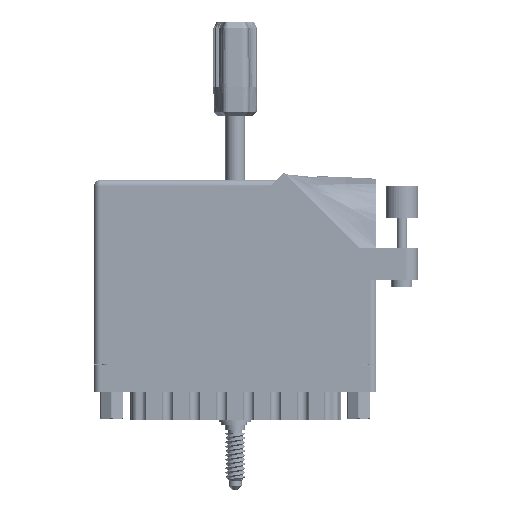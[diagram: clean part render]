
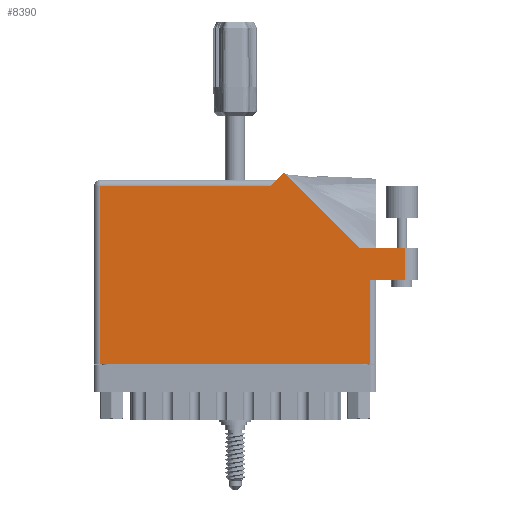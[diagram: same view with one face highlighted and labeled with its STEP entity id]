
A CAD part, front view. The second image highlights one B-rep face of the part: STEP entity #8390.
In plain terms, the highlighted face is planar.
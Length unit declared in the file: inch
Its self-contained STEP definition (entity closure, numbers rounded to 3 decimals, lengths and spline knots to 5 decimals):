
#1445 = ORIENTED_EDGE ( 'NONE', *, *, #68756, .T. ) ;
#1887 = CARTESIAN_POINT ( 'NONE',  ( 2.656, 0.815, 0. ) ) ;
#2625 = EDGE_CURVE ( 'NONE', #33896, #48656, #38547, .T. ) ;
#3944 = ORIENTED_EDGE ( 'NONE', *, *, #40752, .T. ) ;
#4784 = CARTESIAN_POINT ( 'NONE',  ( 3.118, 1.122, 0. ) ) ;
#5384 = DIRECTION ( 'NONE',  ( 0., 0., -1. ) ) ;
#8390 = ADVANCED_FACE ( 'NONE', ( #10046 ), #50888, .F. ) ;
#9209 = VECTOR ( 'NONE', #99094, 39.37008 ) ;
#10046 = FACE_OUTER_BOUND ( 'NONE', #59269, .T. ) ;
#10712 = LINE ( 'NONE', #1887, #82452 ) ;
#11647 = ORIENTED_EDGE ( 'NONE', *, *, #65456, .T. ) ;
#11669 = LINE ( 'NONE', #55826, #53551 ) ;
#15137 = EDGE_CURVE ( 'NONE', #30388, #33896, #11669, .T. ) ;
#16803 = ORIENTED_EDGE ( 'NONE', *, *, #2625, .T. ) ;
#16981 = CARTESIAN_POINT ( 'NONE',  ( 0., 1.713, 0. ) ) ;
#22783 = VECTOR ( 'NONE', #32033, 39.37008 ) ;
#24452 = CARTESIAN_POINT ( 'NONE',  ( 0.062, 0., 0. ) ) ;
#24701 = DIRECTION ( 'NONE',  ( 1., 0., 0. ) ) ;
#25269 = ORIENTED_EDGE ( 'NONE', *, *, #43022, .T. ) ;
#26406 = DIRECTION ( 'NONE',  ( -0.707, -0.707, 0. ) ) ;
#27807 = EDGE_CURVE ( 'NONE', #47507, #82310, #59156, .T. ) ;
#30388 = VERTEX_POINT ( 'NONE', #42587 ) ;
#32033 = DIRECTION ( 'NONE',  ( -1., 0., 0. ) ) ;
#33896 = VERTEX_POINT ( 'NONE', #59352 ) ;
#38547 = LINE ( 'NONE', #94466, #74501 ) ;
#39142 = LINE ( 'NONE', #84057, #9209 ) ;
#40590 = ORIENTED_EDGE ( 'NONE', *, *, #63976, .T. ) ;
#40752 = EDGE_CURVE ( 'NONE', #61225, #71446, #79010, .T. ) ;
#42587 = CARTESIAN_POINT ( 'NONE',  ( 2.656, 0.815, 0. ) ) ;
#43022 = EDGE_CURVE ( 'NONE', #71446, #88513, #39142, .T. ) ;
#44097 = VECTOR ( 'NONE', #95992, 39.37008 ) ;
#45894 = LINE ( 'NONE', #73364, #81697 ) ;
#47507 = VERTEX_POINT ( 'NONE', #72436 ) ;
#48462 = CARTESIAN_POINT ( 'NONE',  ( 2.656, 0., 0. ) ) ;
#48656 = VERTEX_POINT ( 'NONE', #79177 ) ;
#49744 = VECTOR ( 'NONE', #26406, 39.37008 ) ;
#50750 = DIRECTION ( 'NONE',  ( 0., 1., 0. ) ) ;
#50888 = PLANE ( 'NONE',  #83038 ) ;
#53357 = LINE ( 'NONE', #71543, #49744 ) ;
#53551 = VECTOR ( 'NONE', #24701, 39.37008 ) ;
#55826 = CARTESIAN_POINT ( 'NONE',  ( 2.718, 0.815, 0. ) ) ;
#58848 = DIRECTION ( 'NONE',  ( -1., 0., 0. ) ) ;
#59156 = LINE ( 'NONE', #68163, #75819 ) ;
#59269 = EDGE_LOOP ( 'NONE', ( #73333, #16803, #64829, #74927, #40590, #3944, #25269, #11647, #1445 ) ) ;
#59352 = CARTESIAN_POINT ( 'NONE',  ( 2.993, 0.815, 0. ) ) ;
#61171 = DIRECTION ( 'NONE',  ( -0.707, 0.707, 0. ) ) ;
#61225 = VERTEX_POINT ( 'NONE', #90922 ) ;
#63976 = EDGE_CURVE ( 'NONE', #82310, #61225, #53357, .T. ) ;
#64829 = ORIENTED_EDGE ( 'NONE', *, *, #91421, .T. ) ;
#65456 = EDGE_CURVE ( 'NONE', #88513, #72953, #45894, .T. ) ;
#68163 = CARTESIAN_POINT ( 'NONE',  ( 2.55242, 1.122, 0. ) ) ;
#68756 = EDGE_CURVE ( 'NONE', #72953, #30388, #10712, .T. ) ;
#71446 = VERTEX_POINT ( 'NONE', #83401 ) ;
#71543 = CARTESIAN_POINT ( 'NONE',  ( 1.758, 1.775, 0. ) ) ;
#72436 = CARTESIAN_POINT ( 'NONE',  ( 2.55242, 1.122, 0. ) ) ;
#72953 = VERTEX_POINT ( 'NONE', #48462 ) ;
#73333 = ORIENTED_EDGE ( 'NONE', *, *, #15137, .T. ) ;
#73364 = CARTESIAN_POINT ( 'NONE',  ( 0., 0., 0. ) ) ;
#73846 = CARTESIAN_POINT ( 'NONE',  ( 0., 1.775, 0. ) ) ;
#74501 = VECTOR ( 'NONE', #50750, 39.37008 ) ;
#74927 = ORIENTED_EDGE ( 'NONE', *, *, #27807, .T. ) ;
#75120 = LINE ( 'NONE', #4784, #44097 ) ;
#75819 = VECTOR ( 'NONE', #61171, 39.37008 ) ;
#79010 = LINE ( 'NONE', #16981, #22783 ) ;
#79177 = CARTESIAN_POINT ( 'NONE',  ( 2.993, 1.122, 0. ) ) ;
#81697 = VECTOR ( 'NONE', #88062, 39.37008 ) ;
#82310 = VERTEX_POINT ( 'NONE', #92842 ) ;
#82452 = VECTOR ( 'NONE', #93766, 39.37008 ) ;
#83038 = AXIS2_PLACEMENT_3D ( 'NONE', #73846, #5384, #58848 ) ;
#83401 = CARTESIAN_POINT ( 'NONE',  ( 0.062, 1.713, 0. ) ) ;
#84057 = CARTESIAN_POINT ( 'NONE',  ( 0.062, 0., 0. ) ) ;
#88062 = DIRECTION ( 'NONE',  ( 1., 0., 0. ) ) ;
#88513 = VERTEX_POINT ( 'NONE', #24452 ) ;
#90922 = CARTESIAN_POINT ( 'NONE',  ( 1.696, 1.713, 0. ) ) ;
#91421 = EDGE_CURVE ( 'NONE', #48656, #47507, #75120, .T. ) ;
#92842 = CARTESIAN_POINT ( 'NONE',  ( 1.82871, 1.84571, 0. ) ) ;
#93766 = DIRECTION ( 'NONE',  ( 0., 1., 0. ) ) ;
#94466 = CARTESIAN_POINT ( 'NONE',  ( 2.993, 1.122, 0. ) ) ;
#95992 = DIRECTION ( 'NONE',  ( -1., 0., 0. ) ) ;
#99094 = DIRECTION ( 'NONE',  ( 0., -1., 0. ) ) ;
